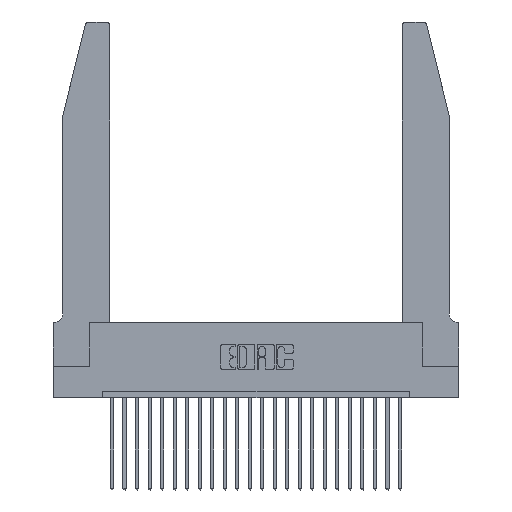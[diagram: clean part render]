
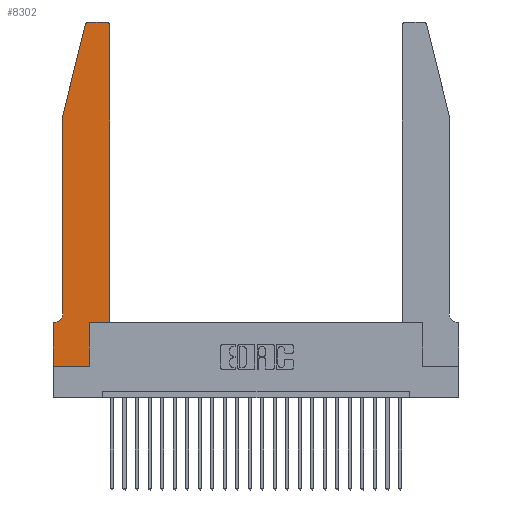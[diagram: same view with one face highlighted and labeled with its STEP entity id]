
A CAD part, top view. The second image highlights one B-rep face of the part: STEP entity #8302.
In plain terms, the highlighted planar face has unit normal (0, 0, 1).
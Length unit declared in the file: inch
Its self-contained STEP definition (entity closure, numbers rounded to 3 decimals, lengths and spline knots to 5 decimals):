
#31 = VERTEX_POINT ( 'NONE', #17310 ) ;
#173 = ORIENTED_EDGE ( 'NONE', *, *, #13800, .T. ) ;
#340 = ORIENTED_EDGE ( 'NONE', *, *, #23249, .T. ) ;
#845 = EDGE_CURVE ( 'NONE', #2462, #2987, #13134, .T. ) ;
#1767 = EDGE_CURVE ( 'NONE', #20206, #19915, #24984, .T. ) ;
#1997 = CARTESIAN_POINT ( 'NONE',  ( 0.0755, 2., 0.37 ) ) ;
#2067 = DIRECTION ( 'NONE',  ( 1., 0., 0. ) ) ;
#2076 = VECTOR ( 'NONE', #21606, 39.37008 ) ;
#2139 = EDGE_CURVE ( 'NONE', #24274, #15169, #2983, .T. ) ;
#2462 = VERTEX_POINT ( 'NONE', #23491 ) ;
#2509 = ORIENTED_EDGE ( 'NONE', *, *, #13692, .T. ) ;
#2983 = LINE ( 'NONE', #14207, #20716 ) ;
#2987 = VERTEX_POINT ( 'NONE', #1997 ) ;
#3059 = LINE ( 'NONE', #14334, #11296 ) ;
#3418 = LINE ( 'NONE', #25208, #8342 ) ;
#3953 = DIRECTION ( 'NONE',  ( 1., 0., 0. ) ) ;
#3997 = EDGE_CURVE ( 'NONE', #19915, #19374, #12046, .T. ) ;
#4091 = CARTESIAN_POINT ( 'NONE',  ( 0.2605, 2.75, 0.37 ) ) ;
#4561 = CARTESIAN_POINT ( 'NONE',  ( 0.0055, 0.35, 0.37 ) ) ;
#4957 = CARTESIAN_POINT ( 'NONE',  ( 0.0755, 0.42, 0.37 ) ) ;
#5025 = ORIENTED_EDGE ( 'NONE', *, *, #18898, .T. ) ;
#5448 = CARTESIAN_POINT ( 'NONE',  ( 0., 0., 0.37 ) ) ;
#5497 = ORIENTED_EDGE ( 'NONE', *, *, #23555, .T. ) ;
#5534 = EDGE_LOOP ( 'NONE', ( #24344, #173, #23802, #25114, #340, #14029, #5497, #2509, #7494, #5025, #13782, #6173 ) ) ;
#5752 = AXIS2_PLACEMENT_3D ( 'NONE', #15602, #20806, #3953 ) ;
#5878 = DIRECTION ( 'NONE',  ( -1., 0., 0. ) ) ;
#6173 = ORIENTED_EDGE ( 'NONE', *, *, #1767, .T. ) ;
#6814 = VECTOR ( 'NONE', #15441, 39.37008 ) ;
#6837 = CARTESIAN_POINT ( 'NONE',  ( 0.284, 2.75, 0.37 ) ) ;
#6853 = VECTOR ( 'NONE', #5878, 39.37008 ) ;
#7467 = CARTESIAN_POINT ( 'NONE',  ( 0.4505, 2.72, 0.37 ) ) ;
#7494 = ORIENTED_EDGE ( 'NONE', *, *, #23751, .T. ) ;
#7738 = LINE ( 'NONE', #23038, #6814 ) ;
#8302 = ADVANCED_FACE ( 'NONE', ( #20650 ), #20057, .T. ) ;
#8342 = VECTOR ( 'NONE', #2067, 39.37008 ) ;
#8510 = DIRECTION ( 'NONE',  ( -0.239, -0.971, 0. ) ) ;
#9141 = CARTESIAN_POINT ( 'NONE',  ( 0.0055, 0.42, 0.37 ) ) ;
#10513 = DIRECTION ( 'NONE',  ( -1., 0., 0. ) ) ;
#10525 = DIRECTION ( 'NONE',  ( 1., 0., 0. ) ) ;
#10659 = DIRECTION ( 'NONE',  ( 0., -1., 0. ) ) ;
#11012 = CARTESIAN_POINT ( 'NONE',  ( 0.2865, 0.35, 0.37 ) ) ;
#11296 = VECTOR ( 'NONE', #24282, 39.37008 ) ;
#12046 = LINE ( 'NONE', #4091, #6853 ) ;
#12211 = EDGE_CURVE ( 'NONE', #18308, #20206, #3059, .T. ) ;
#12422 = CARTESIAN_POINT ( 'NONE',  ( 0.4205, 2.72, 0.37 ) ) ;
#12437 = CARTESIAN_POINT ( 'NONE',  ( 0., 0., 0.37 ) ) ;
#13134 = LINE ( 'NONE', #22100, #23202 ) ;
#13692 = EDGE_CURVE ( 'NONE', #15645, #31, #15508, .T. ) ;
#13782 = ORIENTED_EDGE ( 'NONE', *, *, #12211, .T. ) ;
#13800 = EDGE_CURVE ( 'NONE', #19374, #2462, #21320, .T. ) ;
#14029 = ORIENTED_EDGE ( 'NONE', *, *, #2139, .T. ) ;
#14207 = CARTESIAN_POINT ( 'NONE',  ( 0.0755, 0.35, 0.37 ) ) ;
#14334 = CARTESIAN_POINT ( 'NONE',  ( 0.4505, 0.35, 0.37 ) ) ;
#14409 = DIRECTION ( 'NONE',  ( 1., 0., 0. ) ) ;
#14788 = LINE ( 'NONE', #11012, #19416 ) ;
#15169 = VERTEX_POINT ( 'NONE', #24238 ) ;
#15441 = DIRECTION ( 'NONE',  ( 0., -1., 0. ) ) ;
#15466 = CARTESIAN_POINT ( 'NONE',  ( 0.2865, 0.35, 0.37 ) ) ;
#15508 = LINE ( 'NONE', #22948, #2076 ) ;
#15602 = CARTESIAN_POINT ( 'NONE',  ( 0.284, 2.72, 0.37 ) ) ;
#15645 = VERTEX_POINT ( 'NONE', #5448 ) ;
#16653 = VERTEX_POINT ( 'NONE', #4957 ) ;
#16713 = AXIS2_PLACEMENT_3D ( 'NONE', #12422, #18529, #14409 ) ;
#17310 = CARTESIAN_POINT ( 'NONE',  ( 0.2865, 0., 0.37 ) ) ;
#17405 = CARTESIAN_POINT ( 'NONE',  ( 0.4205, 2.75, 0.37 ) ) ;
#18308 = VERTEX_POINT ( 'NONE', #23407 ) ;
#18326 = CARTESIAN_POINT ( 'NONE',  ( 0., 0.35, 0.37 ) ) ;
#18529 = DIRECTION ( 'NONE',  ( 0., 0., 1. ) ) ;
#18542 = DIRECTION ( 'NONE',  ( 0., 1., 0. ) ) ;
#18898 = EDGE_CURVE ( 'NONE', #23304, #18308, #3418, .T. ) ;
#19374 = VERTEX_POINT ( 'NONE', #6837 ) ;
#19410 = CIRCLE ( 'NONE', #22894, 0.07 ) ;
#19416 = VECTOR ( 'NONE', #18542, 39.37008 ) ;
#19693 = VECTOR ( 'NONE', #10659, 39.37008 ) ;
#19915 = VERTEX_POINT ( 'NONE', #17405 ) ;
#20057 = PLANE ( 'NONE',  #20120 ) ;
#20120 = AXIS2_PLACEMENT_3D ( 'NONE', #18326, #22268, #10525 ) ;
#20206 = VERTEX_POINT ( 'NONE', #7467 ) ;
#20650 = FACE_OUTER_BOUND ( 'NONE', #5534, .T. ) ;
#20716 = VECTOR ( 'NONE', #10513, 39.37008 ) ;
#20806 = DIRECTION ( 'NONE',  ( 0., 0., 1. ) ) ;
#21320 = CIRCLE ( 'NONE', #5752, 0.03 ) ;
#21606 = DIRECTION ( 'NONE',  ( 1., 0., 0. ) ) ;
#22100 = CARTESIAN_POINT ( 'NONE',  ( 0.0755, 2., 0.37 ) ) ;
#22268 = DIRECTION ( 'NONE',  ( 0., 0., 1. ) ) ;
#22827 = DIRECTION ( 'NONE',  ( -1., 0., 0. ) ) ;
#22894 = AXIS2_PLACEMENT_3D ( 'NONE', #9141, #22900, #22827 ) ;
#22900 = DIRECTION ( 'NONE',  ( 0., 0., -1. ) ) ;
#22948 = CARTESIAN_POINT ( 'NONE',  ( 0., 0., 0.37 ) ) ;
#23038 = CARTESIAN_POINT ( 'NONE',  ( 0.0755, 2., 0.37 ) ) ;
#23202 = VECTOR ( 'NONE', #8510, 39.37008 ) ;
#23249 = EDGE_CURVE ( 'NONE', #16653, #24274, #19410, .T. ) ;
#23304 = VERTEX_POINT ( 'NONE', #15466 ) ;
#23407 = CARTESIAN_POINT ( 'NONE',  ( 0.4505, 0.35, 0.37 ) ) ;
#23491 = CARTESIAN_POINT ( 'NONE',  ( 0.25487, 2.72718, 0.37 ) ) ;
#23555 = EDGE_CURVE ( 'NONE', #15169, #15645, #23603, .T. ) ;
#23603 = LINE ( 'NONE', #12437, #19693 ) ;
#23751 = EDGE_CURVE ( 'NONE', #31, #23304, #14788, .T. ) ;
#23802 = ORIENTED_EDGE ( 'NONE', *, *, #845, .T. ) ;
#24238 = CARTESIAN_POINT ( 'NONE',  ( 0., 0.35, 0.37 ) ) ;
#24274 = VERTEX_POINT ( 'NONE', #4561 ) ;
#24282 = DIRECTION ( 'NONE',  ( 0., 1., 0. ) ) ;
#24344 = ORIENTED_EDGE ( 'NONE', *, *, #3997, .T. ) ;
#24562 = EDGE_CURVE ( 'NONE', #2987, #16653, #7738, .T. ) ;
#24984 = CIRCLE ( 'NONE', #16713, 0.03 ) ;
#25114 = ORIENTED_EDGE ( 'NONE', *, *, #24562, .T. ) ;
#25208 = CARTESIAN_POINT ( 'NONE',  ( 0.4505, 0.35, 0.37 ) ) ;
